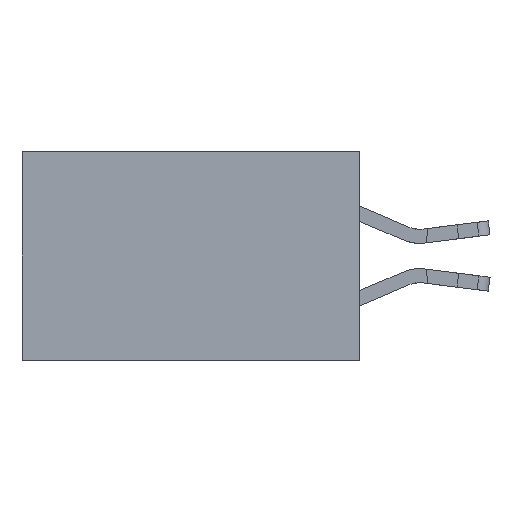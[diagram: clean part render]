
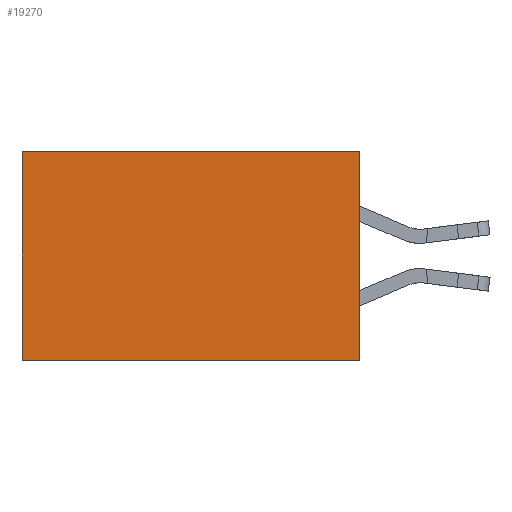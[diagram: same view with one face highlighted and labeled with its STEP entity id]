
A CAD part, left-side view. The second image highlights one B-rep face of the part: STEP entity #19270.
In plain terms, the highlighted planar face has unit normal (-1, 0, 0).
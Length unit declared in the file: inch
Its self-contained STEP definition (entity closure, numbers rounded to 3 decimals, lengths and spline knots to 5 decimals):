
#521 = EDGE_CURVE ( 'NONE', #5235, #30942, #22453, .T. ) ;
#1504 = PLANE ( 'NONE',  #14075 ) ;
#1594 = CARTESIAN_POINT ( 'NONE',  ( 0.2875, 0.6, -0.37 ) ) ;
#2899 = ORIENTED_EDGE ( 'NONE', *, *, #34528, .T. ) ;
#3931 = VERTEX_POINT ( 'NONE', #1594 ) ;
#4780 = LINE ( 'NONE', #32181, #20794 ) ;
#5235 = VERTEX_POINT ( 'NONE', #21974 ) ;
#5626 = VECTOR ( 'NONE', #13761, 39.37008 ) ;
#6346 = VECTOR ( 'NONE', #29301, 39.37008 ) ;
#6461 = ORIENTED_EDGE ( 'NONE', *, *, #20702, .T. ) ;
#6865 = CARTESIAN_POINT ( 'NONE',  ( 0.2875, 0., 0. ) ) ;
#7393 = EDGE_CURVE ( 'NONE', #30942, #3931, #15293, .T. ) ;
#9223 = ORIENTED_EDGE ( 'NONE', *, *, #521, .F. ) ;
#9377 = DIRECTION ( 'NONE',  ( 0., 0., -1. ) ) ;
#12138 = DIRECTION ( 'NONE',  ( 0., 0., -1. ) ) ;
#12717 = VECTOR ( 'NONE', #9377, 39.37008 ) ;
#13477 = CARTESIAN_POINT ( 'NONE',  ( 0.2875, 0.6, 0. ) ) ;
#13761 = DIRECTION ( 'NONE',  ( 0., 1., 0. ) ) ;
#14075 = AXIS2_PLACEMENT_3D ( 'NONE', #6865, #33940, #12138 ) ;
#14298 = EDGE_LOOP ( 'NONE', ( #2899, #31572, #9223, #6461 ) ) ;
#15202 = VERTEX_POINT ( 'NONE', #13477 ) ;
#15293 = LINE ( 'NONE', #26857, #5626 ) ;
#19270 = ADVANCED_FACE ( 'NONE', ( #26387 ), #1504, .F. ) ;
#20702 = EDGE_CURVE ( 'NONE', #5235, #15202, #4780, .T. ) ;
#20794 = VECTOR ( 'NONE', #21501, 39.37008 ) ;
#21501 = DIRECTION ( 'NONE',  ( 0., 1., 0. ) ) ;
#21974 = CARTESIAN_POINT ( 'NONE',  ( 0.2875, 0., 0. ) ) ;
#22453 = LINE ( 'NONE', #25971, #12717 ) ;
#23233 = LINE ( 'NONE', #26554, #6346 ) ;
#25971 = CARTESIAN_POINT ( 'NONE',  ( 0.2875, 0., 0. ) ) ;
#26387 = FACE_OUTER_BOUND ( 'NONE', #14298, .T. ) ;
#26554 = CARTESIAN_POINT ( 'NONE',  ( 0.2875, 0.6, 0. ) ) ;
#26857 = CARTESIAN_POINT ( 'NONE',  ( 0.2875, 0., -0.37 ) ) ;
#27533 = CARTESIAN_POINT ( 'NONE',  ( 0.2875, 0., -0.37 ) ) ;
#29301 = DIRECTION ( 'NONE',  ( 0., 0., -1. ) ) ;
#30942 = VERTEX_POINT ( 'NONE', #27533 ) ;
#31572 = ORIENTED_EDGE ( 'NONE', *, *, #7393, .F. ) ;
#32181 = CARTESIAN_POINT ( 'NONE',  ( 0.2875, 0., 0. ) ) ;
#33940 = DIRECTION ( 'NONE',  ( 1., 0., 0. ) ) ;
#34528 = EDGE_CURVE ( 'NONE', #15202, #3931, #23233, .T. ) ;
